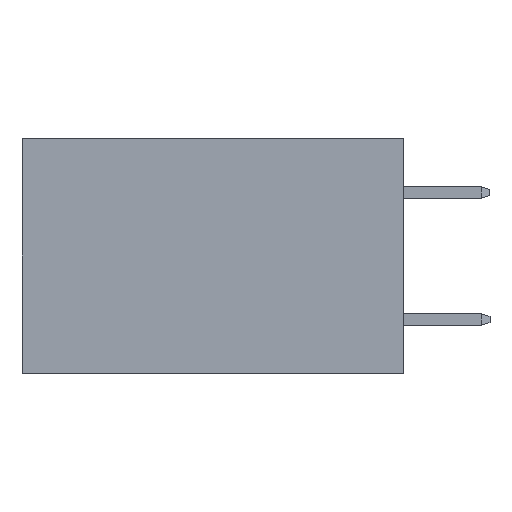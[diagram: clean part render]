
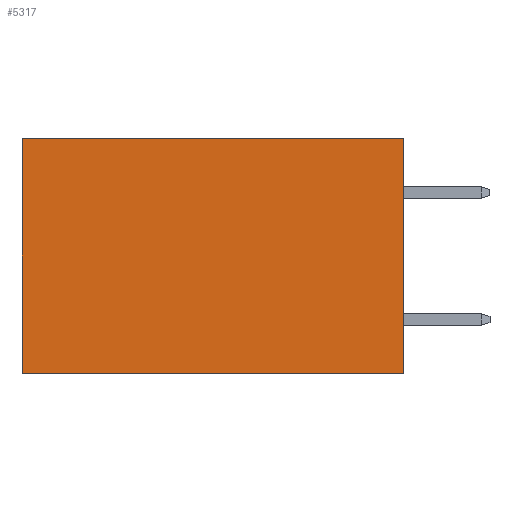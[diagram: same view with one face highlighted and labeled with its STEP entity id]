
A CAD part, left-side view. The second image highlights one B-rep face of the part: STEP entity #5317.
In plain terms, the highlighted planar face has unit normal (-1, 0, 0).
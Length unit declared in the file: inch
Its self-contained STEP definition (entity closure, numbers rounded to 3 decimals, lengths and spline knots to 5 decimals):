
#146 = LINE ( 'NONE', #3666, #9278 ) ;
#323 = CARTESIAN_POINT ( 'NONE',  ( 0.2875, 0.6, 0. ) ) ;
#341 = EDGE_CURVE ( 'NONE', #5558, #5802, #6580, .T. ) ;
#835 = DIRECTION ( 'NONE',  ( 0., 0., -1. ) ) ;
#1309 = VERTEX_POINT ( 'NONE', #7811 ) ;
#1924 = CARTESIAN_POINT ( 'NONE',  ( 0.2875, 0., -0.37 ) ) ;
#1974 = VECTOR ( 'NONE', #835, 39.37008 ) ;
#1996 = AXIS2_PLACEMENT_3D ( 'NONE', #7339, #3081, #3736 ) ;
#2006 = CARTESIAN_POINT ( 'NONE',  ( 0.2875, 0., -0.37 ) ) ;
#2103 = ORIENTED_EDGE ( 'NONE', *, *, #4083, .T. ) ;
#2440 = PLANE ( 'NONE',  #1996 ) ;
#2506 = VECTOR ( 'NONE', #8682, 39.37008 ) ;
#2975 = ORIENTED_EDGE ( 'NONE', *, *, #341, .T. ) ;
#2990 = CARTESIAN_POINT ( 'NONE',  ( 0.2875, 0., 0. ) ) ;
#3081 = DIRECTION ( 'NONE',  ( 1., 0., 0. ) ) ;
#3118 = VECTOR ( 'NONE', #3479, 39.37008 ) ;
#3479 = DIRECTION ( 'NONE',  ( 0., 1., 0. ) ) ;
#3666 = CARTESIAN_POINT ( 'NONE',  ( 0.2875, 0., 0. ) ) ;
#3736 = DIRECTION ( 'NONE',  ( 0., 0., -1. ) ) ;
#4083 = EDGE_CURVE ( 'NONE', #5802, #1309, #5845, .T. ) ;
#4184 = VERTEX_POINT ( 'NONE', #1924 ) ;
#5162 = FACE_OUTER_BOUND ( 'NONE', #8517, .T. ) ;
#5317 = ADVANCED_FACE ( 'NONE', ( #5162 ), #2440, .F. ) ;
#5558 = VERTEX_POINT ( 'NONE', #7276 ) ;
#5802 = VERTEX_POINT ( 'NONE', #323 ) ;
#5845 = LINE ( 'NONE', #8692, #1974 ) ;
#6034 = ORIENTED_EDGE ( 'NONE', *, *, #8383, .F. ) ;
#6422 = ORIENTED_EDGE ( 'NONE', *, *, #6625, .F. ) ;
#6580 = LINE ( 'NONE', #2990, #2506 ) ;
#6625 = EDGE_CURVE ( 'NONE', #5558, #4184, #146, .T. ) ;
#6984 = LINE ( 'NONE', #2006, #3118 ) ;
#7223 = DIRECTION ( 'NONE',  ( 0., 0., -1. ) ) ;
#7276 = CARTESIAN_POINT ( 'NONE',  ( 0.2875, 0., 0. ) ) ;
#7339 = CARTESIAN_POINT ( 'NONE',  ( 0.2875, 0., 0. ) ) ;
#7811 = CARTESIAN_POINT ( 'NONE',  ( 0.2875, 0.6, -0.37 ) ) ;
#8383 = EDGE_CURVE ( 'NONE', #4184, #1309, #6984, .T. ) ;
#8517 = EDGE_LOOP ( 'NONE', ( #2103, #6034, #6422, #2975 ) ) ;
#8682 = DIRECTION ( 'NONE',  ( 0., 1., 0. ) ) ;
#8692 = CARTESIAN_POINT ( 'NONE',  ( 0.2875, 0.6, 0. ) ) ;
#9278 = VECTOR ( 'NONE', #7223, 39.37008 ) ;
